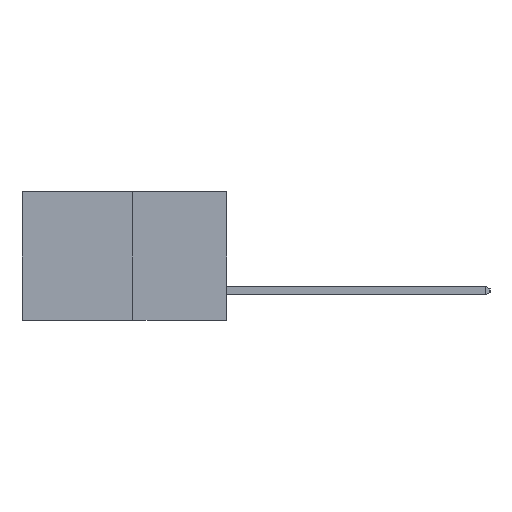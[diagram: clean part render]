
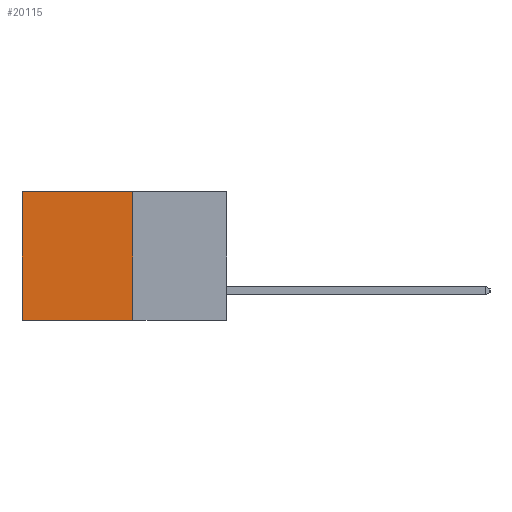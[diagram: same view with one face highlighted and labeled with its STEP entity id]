
A CAD part, left-side view. The second image highlights one B-rep face of the part: STEP entity #20115.
In plain terms, the highlighted planar face has unit normal (-1, 0, 0).
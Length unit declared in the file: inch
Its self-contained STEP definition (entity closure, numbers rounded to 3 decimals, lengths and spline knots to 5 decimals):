
#450 = ORIENTED_EDGE ( 'NONE', *, *, #7793, .F. ) ;
#956 = AXIS2_PLACEMENT_3D ( 'NONE', #9041, #12337, #2340 ) ;
#2340 = DIRECTION ( 'NONE',  ( 0., 0., -1. ) ) ;
#3491 = CARTESIAN_POINT ( 'NONE',  ( 0.277, 0.27, 0. ) ) ;
#4828 = VECTOR ( 'NONE', #17545, 39.37008 ) ;
#4878 = CARTESIAN_POINT ( 'NONE',  ( 0.277, 0.59, -0.37 ) ) ;
#5977 = CARTESIAN_POINT ( 'NONE',  ( 0.277, 0.27, -0.37 ) ) ;
#6474 = FACE_OUTER_BOUND ( 'NONE', #19257, .T. ) ;
#6575 = DIRECTION ( 'NONE',  ( 0., 0., -1. ) ) ;
#6735 = ORIENTED_EDGE ( 'NONE', *, *, #18302, .F. ) ;
#7793 = EDGE_CURVE ( 'NONE', #18318, #14677, #13645, .T. ) ;
#8307 = LINE ( 'NONE', #3491, #12670 ) ;
#9041 = CARTESIAN_POINT ( 'NONE',  ( 0.277, 0.27, -0.37 ) ) ;
#9151 = LINE ( 'NONE', #15016, #17283 ) ;
#10161 = CARTESIAN_POINT ( 'NONE',  ( 0.277, 0.59, 0. ) ) ;
#10211 = CARTESIAN_POINT ( 'NONE',  ( 0.277, 0.27, 0. ) ) ;
#10682 = ORIENTED_EDGE ( 'NONE', *, *, #17560, .T. ) ;
#11490 = VECTOR ( 'NONE', #6575, 39.37008 ) ;
#11507 = ORIENTED_EDGE ( 'NONE', *, *, #12290, .T. ) ;
#12290 = EDGE_CURVE ( 'NONE', #18318, #16817, #8307, .T. ) ;
#12337 = DIRECTION ( 'NONE',  ( 1., 0., 0. ) ) ;
#12670 = VECTOR ( 'NONE', #13485, 39.37008 ) ;
#13039 = PLANE ( 'NONE',  #956 ) ;
#13485 = DIRECTION ( 'NONE',  ( 0., 1., 0. ) ) ;
#13645 = LINE ( 'NONE', #17571, #4828 ) ;
#14677 = VERTEX_POINT ( 'NONE', #5977 ) ;
#15016 = CARTESIAN_POINT ( 'NONE',  ( 0.277, 0.27, -0.37 ) ) ;
#15598 = VERTEX_POINT ( 'NONE', #20031 ) ;
#16635 = DIRECTION ( 'NONE',  ( 0., 1., 0. ) ) ;
#16817 = VERTEX_POINT ( 'NONE', #10161 ) ;
#17283 = VECTOR ( 'NONE', #16635, 39.37008 ) ;
#17545 = DIRECTION ( 'NONE',  ( 0., 0., -1. ) ) ;
#17560 = EDGE_CURVE ( 'NONE', #16817, #15598, #20066, .T. ) ;
#17571 = CARTESIAN_POINT ( 'NONE',  ( 0.277, 0.27, -0.37 ) ) ;
#18302 = EDGE_CURVE ( 'NONE', #14677, #15598, #9151, .T. ) ;
#18318 = VERTEX_POINT ( 'NONE', #10211 ) ;
#19257 = EDGE_LOOP ( 'NONE', ( #10682, #6735, #450, #11507 ) ) ;
#20031 = CARTESIAN_POINT ( 'NONE',  ( 0.277, 0.59, -0.37 ) ) ;
#20066 = LINE ( 'NONE', #4878, #11490 ) ;
#20115 = ADVANCED_FACE ( 'NONE', ( #6474 ), #13039, .F. ) ;
